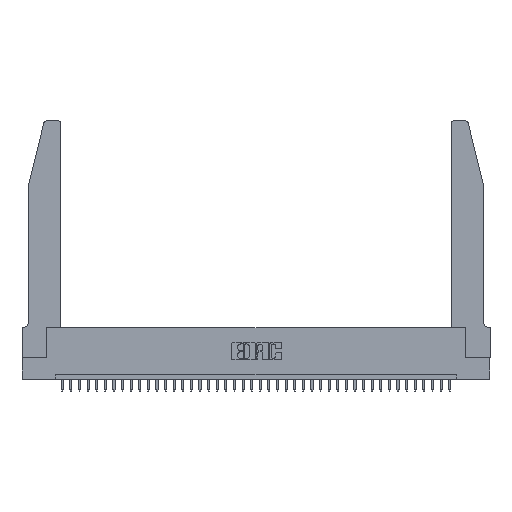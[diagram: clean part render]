
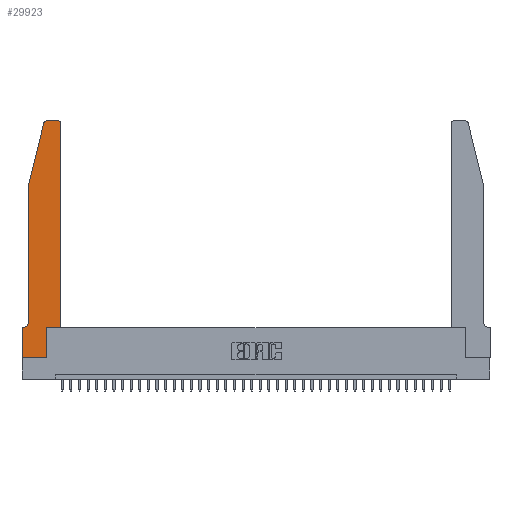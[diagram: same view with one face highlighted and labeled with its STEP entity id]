
A CAD part, top view. The second image highlights one B-rep face of the part: STEP entity #29923.
In plain terms, the highlighted planar face has unit normal (0, 0, 1).
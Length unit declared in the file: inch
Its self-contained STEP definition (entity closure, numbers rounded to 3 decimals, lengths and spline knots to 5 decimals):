
#401 = LINE ( 'NONE', #35082, #11249 ) ;
#802 = AXIS2_PLACEMENT_3D ( 'NONE', #26451, #17277, #20035 ) ;
#917 = CARTESIAN_POINT ( 'NONE',  ( 0.0755, 0.35, 0.37 ) ) ;
#1106 = VERTEX_POINT ( 'NONE', #22064 ) ;
#2091 = LINE ( 'NONE', #16631, #23612 ) ;
#2343 = CARTESIAN_POINT ( 'NONE',  ( 0.2865, 0., 0.37 ) ) ;
#2377 = DIRECTION ( 'NONE',  ( 0., 0., 1. ) ) ;
#2539 = CARTESIAN_POINT ( 'NONE',  ( 0.4505, 0.35, 0.37 ) ) ;
#2876 = PLANE ( 'NONE',  #12979 ) ;
#2889 = CARTESIAN_POINT ( 'NONE',  ( 0.25487, 2.72718, 0.37 ) ) ;
#3024 = CARTESIAN_POINT ( 'NONE',  ( 0.0755, 2., 0.37 ) ) ;
#3119 = CARTESIAN_POINT ( 'NONE',  ( 0., 0., 0.37 ) ) ;
#3262 = LINE ( 'NONE', #917, #10291 ) ;
#3273 = LINE ( 'NONE', #3119, #20184 ) ;
#3321 = EDGE_CURVE ( 'NONE', #16531, #1106, #2091, .T. ) ;
#3440 = VERTEX_POINT ( 'NONE', #26680 ) ;
#3547 = LINE ( 'NONE', #2539, #27509 ) ;
#4293 = CARTESIAN_POINT ( 'NONE',  ( 0.4205, 2.75, 0.37 ) ) ;
#4379 = CARTESIAN_POINT ( 'NONE',  ( 0.4505, 0.35, 0.37 ) ) ;
#4539 = ORIENTED_EDGE ( 'NONE', *, *, #21953, .T. ) ;
#4670 = EDGE_CURVE ( 'NONE', #22336, #4780, #7058, .T. ) ;
#4780 = VERTEX_POINT ( 'NONE', #35792 ) ;
#4865 = VERTEX_POINT ( 'NONE', #31740 ) ;
#6250 = DIRECTION ( 'NONE',  ( 0., 0., 1. ) ) ;
#6417 = CARTESIAN_POINT ( 'NONE',  ( 0.4505, 0.35, 0.37 ) ) ;
#6676 = VERTEX_POINT ( 'NONE', #13104 ) ;
#6838 = LINE ( 'NONE', #38316, #21840 ) ;
#7058 = LINE ( 'NONE', #3024, #27233 ) ;
#8088 = VERTEX_POINT ( 'NONE', #10668 ) ;
#8223 = ORIENTED_EDGE ( 'NONE', *, *, #36866, .T. ) ;
#8243 = ORIENTED_EDGE ( 'NONE', *, *, #20414, .T. ) ;
#9211 = ORIENTED_EDGE ( 'NONE', *, *, #20362, .T. ) ;
#9659 = CARTESIAN_POINT ( 'NONE',  ( 0.4205, 2.72, 0.37 ) ) ;
#10291 = VECTOR ( 'NONE', #37132, 39.37008 ) ;
#10668 = CARTESIAN_POINT ( 'NONE',  ( 0.0755, 0.42, 0.37 ) ) ;
#10796 = CIRCLE ( 'NONE', #38067, 0.03 ) ;
#11249 = VECTOR ( 'NONE', #20106, 39.37008 ) ;
#12897 = CARTESIAN_POINT ( 'NONE',  ( 0., 0.35, 0.37 ) ) ;
#12979 = AXIS2_PLACEMENT_3D ( 'NONE', #33251, #6250, #36391 ) ;
#13104 = CARTESIAN_POINT ( 'NONE',  ( 0., 0., 0.37 ) ) ;
#14948 = DIRECTION ( 'NONE',  ( -0.239, -0.971, 0. ) ) ;
#15196 = VECTOR ( 'NONE', #25474, 39.37008 ) ;
#15478 = DIRECTION ( 'NONE',  ( 0., -1., 0. ) ) ;
#15604 = ORIENTED_EDGE ( 'NONE', *, *, #3321, .T. ) ;
#15839 = ORIENTED_EDGE ( 'NONE', *, *, #35486, .T. ) ;
#16007 = VECTOR ( 'NONE', #15478, 39.37008 ) ;
#16531 = VERTEX_POINT ( 'NONE', #4293 ) ;
#16631 = CARTESIAN_POINT ( 'NONE',  ( 0.2605, 2.75, 0.37 ) ) ;
#16699 = VERTEX_POINT ( 'NONE', #2343 ) ;
#17277 = DIRECTION ( 'NONE',  ( 0., 0., -1. ) ) ;
#17583 = LINE ( 'NONE', #6417, #15196 ) ;
#17792 = CIRCLE ( 'NONE', #21079, 0.03 ) ;
#19794 = EDGE_CURVE ( 'NONE', #4780, #8088, #25868, .T. ) ;
#20035 = DIRECTION ( 'NONE',  ( -1., 0., 0. ) ) ;
#20049 = VERTEX_POINT ( 'NONE', #12897 ) ;
#20106 = DIRECTION ( 'NONE',  ( 0., -1., 0. ) ) ;
#20184 = VECTOR ( 'NONE', #20937, 39.37008 ) ;
#20320 = CARTESIAN_POINT ( 'NONE',  ( 0.284, 2.72, 0.37 ) ) ;
#20362 = EDGE_CURVE ( 'NONE', #3440, #16531, #17792, .T. ) ;
#20414 = EDGE_CURVE ( 'NONE', #32871, #20049, #3262, .T. ) ;
#20937 = DIRECTION ( 'NONE',  ( 1., 0., 0. ) ) ;
#21079 = AXIS2_PLACEMENT_3D ( 'NONE', #9659, #33710, #24919 ) ;
#21840 = VECTOR ( 'NONE', #29169, 39.37008 ) ;
#21953 = EDGE_CURVE ( 'NONE', #4865, #33700, #17583, .T. ) ;
#22064 = CARTESIAN_POINT ( 'NONE',  ( 0.284, 2.75, 0.37 ) ) ;
#22336 = VERTEX_POINT ( 'NONE', #2889 ) ;
#22354 = ORIENTED_EDGE ( 'NONE', *, *, #36716, .T. ) ;
#22502 = ORIENTED_EDGE ( 'NONE', *, *, #19794, .T. ) ;
#22725 = ORIENTED_EDGE ( 'NONE', *, *, #4670, .T. ) ;
#23475 = DIRECTION ( 'NONE',  ( 0., 1., 0. ) ) ;
#23612 = VECTOR ( 'NONE', #34979, 39.37008 ) ;
#24245 = EDGE_CURVE ( 'NONE', #20049, #6676, #401, .T. ) ;
#24919 = DIRECTION ( 'NONE',  ( 1., 0., 0. ) ) ;
#25474 = DIRECTION ( 'NONE',  ( 1., 0., 0. ) ) ;
#25723 = ORIENTED_EDGE ( 'NONE', *, *, #33784, .T. ) ;
#25868 = LINE ( 'NONE', #36325, #16007 ) ;
#26293 = ORIENTED_EDGE ( 'NONE', *, *, #33842, .T. ) ;
#26451 = CARTESIAN_POINT ( 'NONE',  ( 0.0055, 0.42, 0.37 ) ) ;
#26623 = DIRECTION ( 'NONE',  ( 1., 0., 0. ) ) ;
#26680 = CARTESIAN_POINT ( 'NONE',  ( 0.4505, 2.72, 0.37 ) ) ;
#27233 = VECTOR ( 'NONE', #14948, 39.37008 ) ;
#27509 = VECTOR ( 'NONE', #23475, 39.37008 ) ;
#29169 = DIRECTION ( 'NONE',  ( 0., 1., 0. ) ) ;
#29923 = ADVANCED_FACE ( 'NONE', ( #36482 ), #2876, .T. ) ;
#31176 = CIRCLE ( 'NONE', #802, 0.07 ) ;
#31288 = EDGE_LOOP ( 'NONE', ( #15604, #22354, #22725, #22502, #15839, #8243, #32480, #8223, #25723, #4539, #26293, #9211 ) ) ;
#31592 = CARTESIAN_POINT ( 'NONE',  ( 0.0055, 0.35, 0.37 ) ) ;
#31740 = CARTESIAN_POINT ( 'NONE',  ( 0.2865, 0.35, 0.37 ) ) ;
#32480 = ORIENTED_EDGE ( 'NONE', *, *, #24245, .T. ) ;
#32871 = VERTEX_POINT ( 'NONE', #31592 ) ;
#33251 = CARTESIAN_POINT ( 'NONE',  ( 0., 0.35, 0.37 ) ) ;
#33700 = VERTEX_POINT ( 'NONE', #4379 ) ;
#33710 = DIRECTION ( 'NONE',  ( 0., 0., 1. ) ) ;
#33784 = EDGE_CURVE ( 'NONE', #16699, #4865, #6838, .T. ) ;
#33842 = EDGE_CURVE ( 'NONE', #33700, #3440, #3547, .T. ) ;
#34979 = DIRECTION ( 'NONE',  ( -1., 0., 0. ) ) ;
#35082 = CARTESIAN_POINT ( 'NONE',  ( 0., 0., 0.37 ) ) ;
#35486 = EDGE_CURVE ( 'NONE', #8088, #32871, #31176, .T. ) ;
#35792 = CARTESIAN_POINT ( 'NONE',  ( 0.0755, 2., 0.37 ) ) ;
#36325 = CARTESIAN_POINT ( 'NONE',  ( 0.0755, 2., 0.37 ) ) ;
#36391 = DIRECTION ( 'NONE',  ( 1., 0., 0. ) ) ;
#36482 = FACE_OUTER_BOUND ( 'NONE', #31288, .T. ) ;
#36716 = EDGE_CURVE ( 'NONE', #1106, #22336, #10796, .T. ) ;
#36866 = EDGE_CURVE ( 'NONE', #6676, #16699, #3273, .T. ) ;
#37132 = DIRECTION ( 'NONE',  ( -1., 0., 0. ) ) ;
#38067 = AXIS2_PLACEMENT_3D ( 'NONE', #20320, #2377, #26623 ) ;
#38316 = CARTESIAN_POINT ( 'NONE',  ( 0.2865, 0.35, 0.37 ) ) ;
